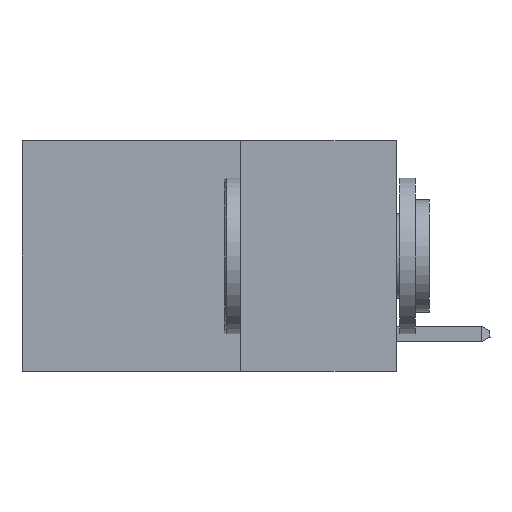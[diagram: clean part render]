
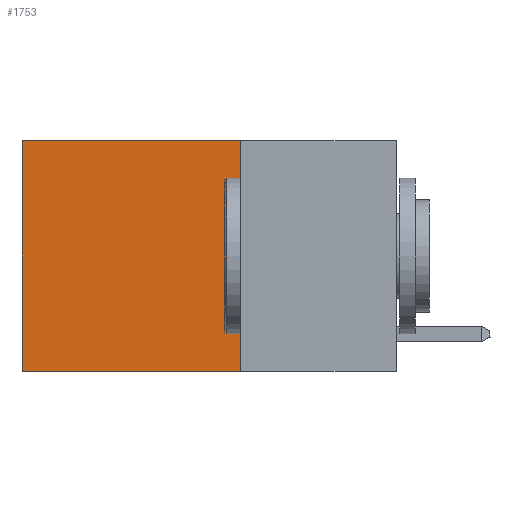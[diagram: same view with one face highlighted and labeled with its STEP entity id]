
A CAD part, left-side view. The second image highlights one B-rep face of the part: STEP entity #1753.
In plain terms, the highlighted planar face has unit normal (-1, 0, 0).
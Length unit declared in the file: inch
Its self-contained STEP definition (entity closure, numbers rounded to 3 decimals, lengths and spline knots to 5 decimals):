
#602 = EDGE_LOOP ( 'NONE', ( #1582, #8254, #6046, #10164 ) ) ;
#948 = EDGE_CURVE ( 'NONE', #4747, #3458, #1259, .T. ) ;
#989 = CARTESIAN_POINT ( 'NONE',  ( 0.2625, 0.6, 0. ) ) ;
#1026 = CARTESIAN_POINT ( 'NONE',  ( 0.2625, 0.25, 0. ) ) ;
#1259 = LINE ( 'NONE', #6418, #10146 ) ;
#1507 = CARTESIAN_POINT ( 'NONE',  ( 0.2625, 0.25, 0. ) ) ;
#1582 = ORIENTED_EDGE ( 'NONE', *, *, #3805, .T. ) ;
#1753 = ADVANCED_FACE ( 'NONE', ( #4436 ), #6364, .F. ) ;
#1761 = VERTEX_POINT ( 'NONE', #989 ) ;
#2006 = DIRECTION ( 'NONE',  ( 0., 0., -1. ) ) ;
#2073 = DIRECTION ( 'NONE',  ( 0., 1., 0. ) ) ;
#3094 = DIRECTION ( 'NONE',  ( 0., 0., -1. ) ) ;
#3309 = AXIS2_PLACEMENT_3D ( 'NONE', #1026, #7199, #2006 ) ;
#3354 = LINE ( 'NONE', #8191, #9769 ) ;
#3458 = VERTEX_POINT ( 'NONE', #10222 ) ;
#3579 = CARTESIAN_POINT ( 'NONE',  ( 0.2625, 0.25, 0. ) ) ;
#3643 = LINE ( 'NONE', #5839, #5909 ) ;
#3805 = EDGE_CURVE ( 'NONE', #1761, #3458, #3643, .T. ) ;
#3993 = LINE ( 'NONE', #1507, #6234 ) ;
#4436 = FACE_OUTER_BOUND ( 'NONE', #602, .T. ) ;
#4747 = VERTEX_POINT ( 'NONE', #5326 ) ;
#5002 = DIRECTION ( 'NONE',  ( 0., 0., -1. ) ) ;
#5326 = CARTESIAN_POINT ( 'NONE',  ( 0.2625, 0.25, -0.37 ) ) ;
#5839 = CARTESIAN_POINT ( 'NONE',  ( 0.2625, 0.6, 0. ) ) ;
#5909 = VECTOR ( 'NONE', #5002, 39.37008 ) ;
#6046 = ORIENTED_EDGE ( 'NONE', *, *, #10446, .F. ) ;
#6234 = VECTOR ( 'NONE', #7618, 39.37008 ) ;
#6364 = PLANE ( 'NONE',  #3309 ) ;
#6418 = CARTESIAN_POINT ( 'NONE',  ( 0.2625, 0.25, -0.37 ) ) ;
#7199 = DIRECTION ( 'NONE',  ( 1., 0., 0. ) ) ;
#7385 = EDGE_CURVE ( 'NONE', #9169, #1761, #3993, .T. ) ;
#7618 = DIRECTION ( 'NONE',  ( 0., 1., 0. ) ) ;
#8191 = CARTESIAN_POINT ( 'NONE',  ( 0.2625, 0.25, 0. ) ) ;
#8254 = ORIENTED_EDGE ( 'NONE', *, *, #948, .F. ) ;
#9169 = VERTEX_POINT ( 'NONE', #3579 ) ;
#9769 = VECTOR ( 'NONE', #3094, 39.37008 ) ;
#10146 = VECTOR ( 'NONE', #2073, 39.37008 ) ;
#10164 = ORIENTED_EDGE ( 'NONE', *, *, #7385, .T. ) ;
#10222 = CARTESIAN_POINT ( 'NONE',  ( 0.2625, 0.6, -0.37 ) ) ;
#10446 = EDGE_CURVE ( 'NONE', #9169, #4747, #3354, .T. ) ;
